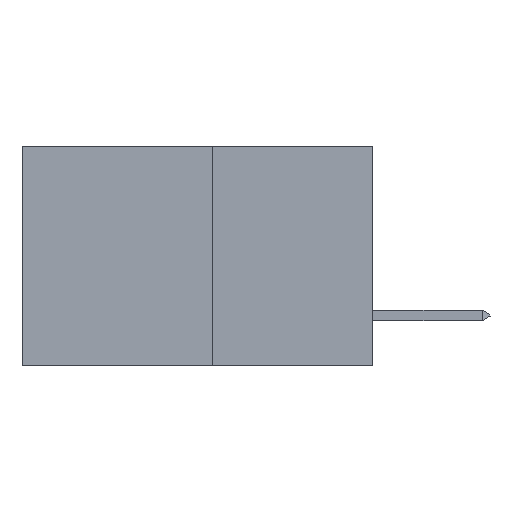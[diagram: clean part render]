
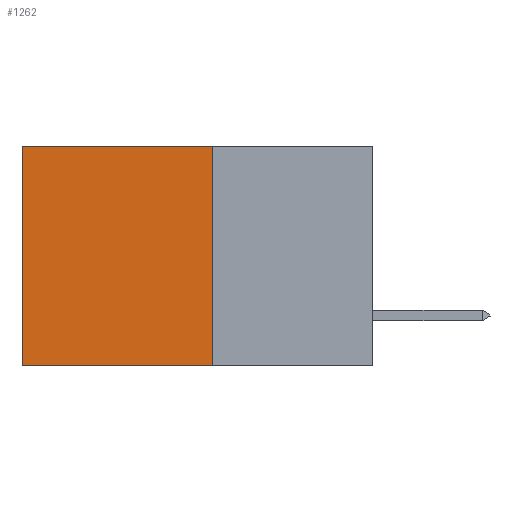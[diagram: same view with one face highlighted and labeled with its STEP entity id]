
A CAD part, left-side view. The second image highlights one B-rep face of the part: STEP entity #1262.
In plain terms, the highlighted planar face has unit normal (-1, 0, 0).
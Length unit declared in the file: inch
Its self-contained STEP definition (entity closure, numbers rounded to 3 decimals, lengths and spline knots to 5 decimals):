
#1262 = ADVANCED_FACE ( 'NONE', ( #14780 ), #14889, .F. ) ;
#1520 = VECTOR ( 'NONE', #13799, 39.37008 ) ;
#2795 = CARTESIAN_POINT ( 'NONE',  ( 0.277, 0.59, -0.37 ) ) ;
#3267 = DIRECTION ( 'NONE',  ( 0., 0., -1. ) ) ;
#3958 = LINE ( 'NONE', #8410, #7811 ) ;
#4477 = DIRECTION ( 'NONE',  ( 0., 1., 0. ) ) ;
#4546 = VERTEX_POINT ( 'NONE', #6821 ) ;
#5587 = DIRECTION ( 'NONE',  ( 0., 1., 0. ) ) ;
#5612 = VECTOR ( 'NONE', #5587, 39.37008 ) ;
#5684 = EDGE_CURVE ( 'NONE', #12641, #7659, #7435, .T. ) ;
#6025 = LINE ( 'NONE', #15568, #5612 ) ;
#6821 = CARTESIAN_POINT ( 'NONE',  ( 0.277, 0.27, -0.37 ) ) ;
#7408 = CARTESIAN_POINT ( 'NONE',  ( 0.277, 0.59, 0. ) ) ;
#7435 = LINE ( 'NONE', #2795, #13652 ) ;
#7568 = CARTESIAN_POINT ( 'NONE',  ( 0.277, 0.27, -0.37 ) ) ;
#7659 = VERTEX_POINT ( 'NONE', #10158 ) ;
#7811 = VECTOR ( 'NONE', #4477, 39.37008 ) ;
#8410 = CARTESIAN_POINT ( 'NONE',  ( 0.277, 0.27, -0.37 ) ) ;
#8496 = CARTESIAN_POINT ( 'NONE',  ( 0.277, 0.27, 0. ) ) ;
#8597 = ORIENTED_EDGE ( 'NONE', *, *, #5684, .T. ) ;
#8670 = ORIENTED_EDGE ( 'NONE', *, *, #8750, .F. ) ;
#8743 = ORIENTED_EDGE ( 'NONE', *, *, #13715, .F. ) ;
#8750 = EDGE_CURVE ( 'NONE', #4546, #7659, #3958, .T. ) ;
#8770 = ORIENTED_EDGE ( 'NONE', *, *, #14685, .T. ) ;
#10158 = CARTESIAN_POINT ( 'NONE',  ( 0.277, 0.59, -0.37 ) ) ;
#11373 = VERTEX_POINT ( 'NONE', #8496 ) ;
#11407 = EDGE_LOOP ( 'NONE', ( #8597, #8670, #8743, #8770 ) ) ;
#11566 = LINE ( 'NONE', #7568, #1520 ) ;
#12162 = AXIS2_PLACEMENT_3D ( 'NONE', #14999, #14730, #15768 ) ;
#12641 = VERTEX_POINT ( 'NONE', #7408 ) ;
#13652 = VECTOR ( 'NONE', #3267, 39.37008 ) ;
#13715 = EDGE_CURVE ( 'NONE', #11373, #4546, #11566, .T. ) ;
#13799 = DIRECTION ( 'NONE',  ( 0., 0., -1. ) ) ;
#14685 = EDGE_CURVE ( 'NONE', #11373, #12641, #6025, .T. ) ;
#14730 = DIRECTION ( 'NONE',  ( 1., 0., 0. ) ) ;
#14780 = FACE_OUTER_BOUND ( 'NONE', #11407, .T. ) ;
#14889 = PLANE ( 'NONE',  #12162 ) ;
#14999 = CARTESIAN_POINT ( 'NONE',  ( 0.277, 0.27, -0.37 ) ) ;
#15568 = CARTESIAN_POINT ( 'NONE',  ( 0.277, 0.27, 0. ) ) ;
#15768 = DIRECTION ( 'NONE',  ( 0., 0., -1. ) ) ;
